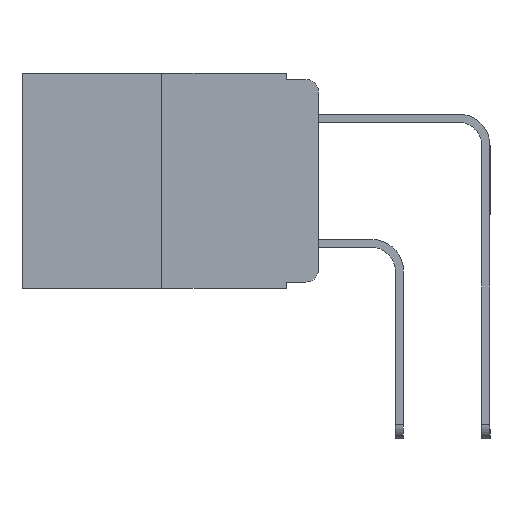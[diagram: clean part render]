
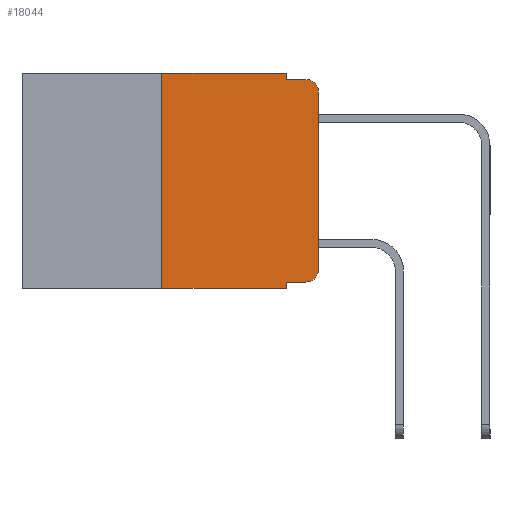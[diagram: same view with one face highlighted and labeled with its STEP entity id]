
A CAD part, left-side view. The second image highlights one B-rep face of the part: STEP entity #18044.
In plain terms, the highlighted planar face has unit normal (-1, 0, 0).
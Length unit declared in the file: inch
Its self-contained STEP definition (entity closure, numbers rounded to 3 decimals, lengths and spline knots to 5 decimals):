
#570 = CIRCLE ( 'NONE', #14194, 0.02 ) ;
#601 = VECTOR ( 'NONE', #19052, 39.37008 ) ;
#931 = VERTEX_POINT ( 'NONE', #19886 ) ;
#975 = VERTEX_POINT ( 'NONE', #20158 ) ;
#2293 = EDGE_CURVE ( 'NONE', #11718, #16149, #12183, .T. ) ;
#3132 = CARTESIAN_POINT ( 'NONE',  ( 0., 0.02, -0.333 ) ) ;
#3791 = EDGE_CURVE ( 'NONE', #931, #16149, #570, .T. ) ;
#3878 = VERTEX_POINT ( 'NONE', #6245 ) ;
#3948 = PLANE ( 'NONE',  #16743 ) ;
#4057 = CARTESIAN_POINT ( 'NONE',  ( 0., 0.02, -0.01 ) ) ;
#4141 = CARTESIAN_POINT ( 'NONE',  ( 0., 0.473, -0.343 ) ) ;
#4353 = CARTESIAN_POINT ( 'NONE',  ( 0., 0.051, -0.01 ) ) ;
#4571 = ORIENTED_EDGE ( 'NONE', *, *, #5294, .T. ) ;
#4578 = CARTESIAN_POINT ( 'NONE',  ( 0., 0.051, -0.333 ) ) ;
#4783 = ORIENTED_EDGE ( 'NONE', *, *, #10915, .F. ) ;
#4852 = VECTOR ( 'NONE', #26657, 39.37008 ) ;
#4854 = ORIENTED_EDGE ( 'NONE', *, *, #27472, .F. ) ;
#5101 = ORIENTED_EDGE ( 'NONE', *, *, #21832, .F. ) ;
#5285 = ORIENTED_EDGE ( 'NONE', *, *, #2293, .F. ) ;
#5294 = EDGE_CURVE ( 'NONE', #14754, #931, #10252, .T. ) ;
#5295 = CARTESIAN_POINT ( 'NONE',  ( 0., 0.25, 0. ) ) ;
#5449 = ORIENTED_EDGE ( 'NONE', *, *, #20434, .F. ) ;
#5570 = LINE ( 'NONE', #7372, #4852 ) ;
#6229 = DIRECTION ( 'NONE',  ( 1., 0., 0. ) ) ;
#6245 = CARTESIAN_POINT ( 'NONE',  ( 0., 0.25, -0.343 ) ) ;
#6346 = ORIENTED_EDGE ( 'NONE', *, *, #18994, .T. ) ;
#7372 = CARTESIAN_POINT ( 'NONE',  ( 0., 0.051, -0.333 ) ) ;
#7707 = DIRECTION ( 'NONE',  ( 0., -1., 0. ) ) ;
#7732 = DIRECTION ( 'NONE',  ( -1., 0., 0. ) ) ;
#8038 = CARTESIAN_POINT ( 'NONE',  ( 0., 0.473, 0. ) ) ;
#8291 = ORIENTED_EDGE ( 'NONE', *, *, #13283, .T. ) ;
#8370 = CARTESIAN_POINT ( 'NONE',  ( 0., 0.473, 0. ) ) ;
#8563 = VERTEX_POINT ( 'NONE', #9959 ) ;
#9803 = ORIENTED_EDGE ( 'NONE', *, *, #3791, .T. ) ;
#9916 = CARTESIAN_POINT ( 'NONE',  ( 0., 0.051, -0.01 ) ) ;
#9959 = CARTESIAN_POINT ( 'NONE',  ( 0., 0.051, 0. ) ) ;
#10164 = CARTESIAN_POINT ( 'NONE',  ( 0., 0.051, 0. ) ) ;
#10204 = VECTOR ( 'NONE', #13088, 39.37008 ) ;
#10248 = DIRECTION ( 'NONE',  ( 0., -1., 0. ) ) ;
#10252 = LINE ( 'NONE', #26535, #25934 ) ;
#10402 = CARTESIAN_POINT ( 'NONE',  ( 0., 0.02, -0.03 ) ) ;
#10915 = EDGE_CURVE ( 'NONE', #12611, #8563, #17257, .T. ) ;
#11089 = VERTEX_POINT ( 'NONE', #4578 ) ;
#11178 = ORIENTED_EDGE ( 'NONE', *, *, #24494, .T. ) ;
#11573 = VECTOR ( 'NONE', #10248, 39.37008 ) ;
#11675 = DIRECTION ( 'NONE',  ( 0., 0., 1. ) ) ;
#11718 = VERTEX_POINT ( 'NONE', #4353 ) ;
#12183 = LINE ( 'NONE', #9916, #27104 ) ;
#12611 = VERTEX_POINT ( 'NONE', #5295 ) ;
#12640 = DIRECTION ( 'NONE',  ( 0., 0., -1. ) ) ;
#12921 = FACE_OUTER_BOUND ( 'NONE', #13313, .T. ) ;
#13088 = DIRECTION ( 'NONE',  ( 0., -1., 0. ) ) ;
#13114 = VECTOR ( 'NONE', #26870, 39.37008 ) ;
#13127 = LINE ( 'NONE', #25410, #601 ) ;
#13283 = EDGE_CURVE ( 'NONE', #23072, #14754, #15141, .T. ) ;
#13313 = EDGE_LOOP ( 'NONE', ( #4571, #9803, #5285, #4854, #4783, #5101, #11178, #5449, #6346, #8291 ) ) ;
#14194 = AXIS2_PLACEMENT_3D ( 'NONE', #10402, #25348, #12640 ) ;
#14520 = LINE ( 'NONE', #10164, #25743 ) ;
#14754 = VERTEX_POINT ( 'NONE', #27052 ) ;
#15141 = CIRCLE ( 'NONE', #21975, 0.02 ) ;
#16149 = VERTEX_POINT ( 'NONE', #4057 ) ;
#16342 = CARTESIAN_POINT ( 'NONE',  ( 0., 0.051, 0. ) ) ;
#16743 = AXIS2_PLACEMENT_3D ( 'NONE', #8370, #6229, #21361 ) ;
#17257 = LINE ( 'NONE', #8038, #11573 ) ;
#18044 = ADVANCED_FACE ( 'NONE', ( #12921 ), #3948, .F. ) ;
#18994 = EDGE_CURVE ( 'NONE', #11089, #23072, #5570, .T. ) ;
#19052 = DIRECTION ( 'NONE',  ( 0., 0., 1. ) ) ;
#19886 = CARTESIAN_POINT ( 'NONE',  ( 0., 0., -0.03 ) ) ;
#20158 = CARTESIAN_POINT ( 'NONE',  ( 0., 0.051, -0.343 ) ) ;
#20434 = EDGE_CURVE ( 'NONE', #11089, #975, #24399, .T. ) ;
#20658 = CARTESIAN_POINT ( 'NONE',  ( 0., 0.02, -0.313 ) ) ;
#21361 = DIRECTION ( 'NONE',  ( 0., 0., -1. ) ) ;
#21620 = LINE ( 'NONE', #4141, #10204 ) ;
#21832 = EDGE_CURVE ( 'NONE', #3878, #12611, #13127, .T. ) ;
#21975 = AXIS2_PLACEMENT_3D ( 'NONE', #20658, #7732, #22768 ) ;
#22768 = DIRECTION ( 'NONE',  ( 0., 0., -1. ) ) ;
#23072 = VERTEX_POINT ( 'NONE', #3132 ) ;
#24399 = LINE ( 'NONE', #16342, #13114 ) ;
#24494 = EDGE_CURVE ( 'NONE', #3878, #975, #21620, .T. ) ;
#25105 = DIRECTION ( 'NONE',  ( 0., 0., -1. ) ) ;
#25348 = DIRECTION ( 'NONE',  ( -1., 0., 0. ) ) ;
#25410 = CARTESIAN_POINT ( 'NONE',  ( 0., 0.25, 0. ) ) ;
#25743 = VECTOR ( 'NONE', #25105, 39.37008 ) ;
#25934 = VECTOR ( 'NONE', #11675, 39.37008 ) ;
#26535 = CARTESIAN_POINT ( 'NONE',  ( 0., 0., 0. ) ) ;
#26657 = DIRECTION ( 'NONE',  ( 0., -1., 0. ) ) ;
#26870 = DIRECTION ( 'NONE',  ( 0., 0., -1. ) ) ;
#27052 = CARTESIAN_POINT ( 'NONE',  ( 0., 0., -0.313 ) ) ;
#27104 = VECTOR ( 'NONE', #7707, 39.37008 ) ;
#27472 = EDGE_CURVE ( 'NONE', #8563, #11718, #14520, .T. ) ;
